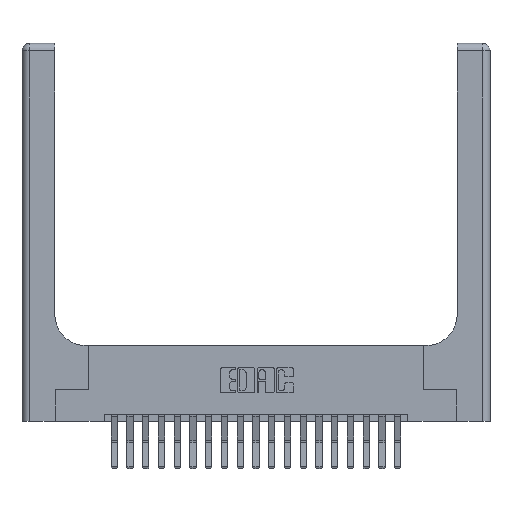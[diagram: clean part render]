
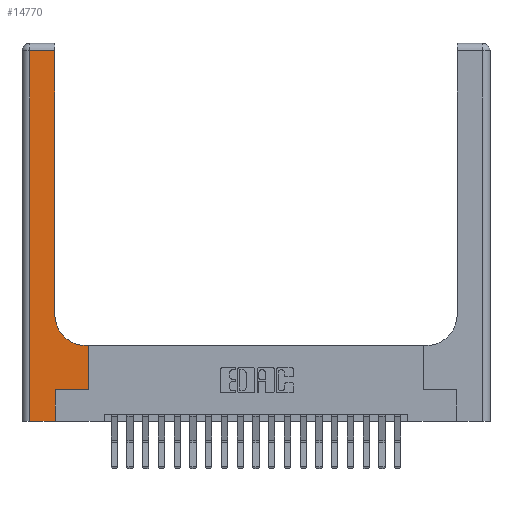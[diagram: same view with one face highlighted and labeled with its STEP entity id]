
A CAD part, top view. The second image highlights one B-rep face of the part: STEP entity #14770.
In plain terms, the highlighted planar face has unit normal (0, 0, 1).
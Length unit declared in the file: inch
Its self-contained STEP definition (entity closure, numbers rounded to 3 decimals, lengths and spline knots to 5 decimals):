
#104 = DIRECTION ( 'NONE',  ( -1., 0., 0. ) ) ;
#171 = AXIS2_PLACEMENT_3D ( 'NONE', #11845, #18023, #13234 ) ;
#428 = AXIS2_PLACEMENT_3D ( 'NONE', #6232, #6744, #3614 ) ;
#624 = PLANE ( 'NONE',  #171 ) ;
#660 = CARTESIAN_POINT ( 'NONE',  ( 0.265, 0., 0.37 ) ) ;
#734 = LINE ( 'NONE', #19692, #10014 ) ;
#1097 = ORIENTED_EDGE ( 'NONE', *, *, #12004, .T. ) ;
#1390 = ORIENTED_EDGE ( 'NONE', *, *, #6338, .T. ) ;
#1741 = CARTESIAN_POINT ( 'NONE',  ( 0.528, 0.6, 0.37 ) ) ;
#2128 = VERTEX_POINT ( 'NONE', #15202 ) ;
#2499 = ORIENTED_EDGE ( 'NONE', *, *, #4910, .T. ) ;
#2816 = ORIENTED_EDGE ( 'NONE', *, *, #12132, .T. ) ;
#3066 = CARTESIAN_POINT ( 'NONE',  ( 0.26, 2.94, 0.37 ) ) ;
#3614 = DIRECTION ( 'NONE',  ( 1., 0., 0. ) ) ;
#3796 = LINE ( 'NONE', #9375, #9843 ) ;
#3816 = ORIENTED_EDGE ( 'NONE', *, *, #19286, .T. ) ;
#4628 = LINE ( 'NONE', #12545, #4862 ) ;
#4636 = LINE ( 'NONE', #17429, #7363 ) ;
#4812 = CARTESIAN_POINT ( 'NONE',  ( 0., 0., 0.37 ) ) ;
#4831 = ORIENTED_EDGE ( 'NONE', *, *, #18948, .T. ) ;
#4835 = DIRECTION ( 'NONE',  ( -1., 0., 0. ) ) ;
#4862 = VECTOR ( 'NONE', #5968, 39.37008 ) ;
#4910 = EDGE_CURVE ( 'NONE', #11582, #2128, #4636, .T. ) ;
#5968 = DIRECTION ( 'NONE',  ( 0., 1., 0. ) ) ;
#6198 = ORIENTED_EDGE ( 'NONE', *, *, #20496, .T. ) ;
#6232 = CARTESIAN_POINT ( 'NONE',  ( 0.51, 0.85, 0.37 ) ) ;
#6338 = EDGE_CURVE ( 'NONE', #17638, #14887, #8106, .T. ) ;
#6652 = VERTEX_POINT ( 'NONE', #9363 ) ;
#6744 = DIRECTION ( 'NONE',  ( 0., 0., -1. ) ) ;
#6790 = LINE ( 'NONE', #19255, #13029 ) ;
#7363 = VECTOR ( 'NONE', #4835, 39.37008 ) ;
#7377 = CARTESIAN_POINT ( 'NONE',  ( 0.265, 0.25, 0.37 ) ) ;
#7416 = EDGE_CURVE ( 'NONE', #7920, #6652, #15059, .T. ) ;
#7920 = VERTEX_POINT ( 'NONE', #18841 ) ;
#8068 = CIRCLE ( 'NONE', #428, 0.25 ) ;
#8106 = LINE ( 'NONE', #11515, #16104 ) ;
#8283 = DIRECTION ( 'NONE',  ( 1., 0., 0. ) ) ;
#9306 = DIRECTION ( 'NONE',  ( 1., 0., 0. ) ) ;
#9363 = CARTESIAN_POINT ( 'NONE',  ( 0.06, 0., 0.37 ) ) ;
#9375 = CARTESIAN_POINT ( 'NONE',  ( 0.265, 0.25, 0.37 ) ) ;
#9843 = VECTOR ( 'NONE', #9306, 39.37008 ) ;
#10014 = VECTOR ( 'NONE', #11834, 39.37008 ) ;
#10081 = VECTOR ( 'NONE', #20060, 39.37008 ) ;
#10682 = CARTESIAN_POINT ( 'NONE',  ( 0.26, 0.85, 0.37 ) ) ;
#10683 = FACE_OUTER_BOUND ( 'NONE', #16678, .T. ) ;
#11515 = CARTESIAN_POINT ( 'NONE',  ( 0.265, 0., 0.37 ) ) ;
#11580 = CARTESIAN_POINT ( 'NONE',  ( 0.06, 3., 0.37 ) ) ;
#11582 = VERTEX_POINT ( 'NONE', #1741 ) ;
#11834 = DIRECTION ( 'NONE',  ( 0., 1., 0. ) ) ;
#11845 = CARTESIAN_POINT ( 'NONE',  ( 0., 3., 0.37 ) ) ;
#12004 = EDGE_CURVE ( 'NONE', #14242, #13864, #4628, .T. ) ;
#12132 = EDGE_CURVE ( 'NONE', #2128, #14242, #8068, .T. ) ;
#12137 = VERTEX_POINT ( 'NONE', #14777 ) ;
#12167 = ORIENTED_EDGE ( 'NONE', *, *, #15923, .T. ) ;
#12545 = CARTESIAN_POINT ( 'NONE',  ( 0.26, 3., 0.37 ) ) ;
#13029 = VECTOR ( 'NONE', #104, 39.37008 ) ;
#13169 = ORIENTED_EDGE ( 'NONE', *, *, #7416, .T. ) ;
#13234 = DIRECTION ( 'NONE',  ( -1., 0., 0. ) ) ;
#13584 = LINE ( 'NONE', #4812, #14093 ) ;
#13864 = VERTEX_POINT ( 'NONE', #3066 ) ;
#14093 = VECTOR ( 'NONE', #8283, 39.37008 ) ;
#14242 = VERTEX_POINT ( 'NONE', #10682 ) ;
#14770 = ADVANCED_FACE ( 'NONE', ( #10683 ), #624, .F. ) ;
#14777 = CARTESIAN_POINT ( 'NONE',  ( 0.528, 0.25, 0.37 ) ) ;
#14887 = VERTEX_POINT ( 'NONE', #7377 ) ;
#15059 = LINE ( 'NONE', #11580, #10081 ) ;
#15202 = CARTESIAN_POINT ( 'NONE',  ( 0.51, 0.6, 0.37 ) ) ;
#15923 = EDGE_CURVE ( 'NONE', #14887, #12137, #3796, .T. ) ;
#16104 = VECTOR ( 'NONE', #16542, 39.37008 ) ;
#16542 = DIRECTION ( 'NONE',  ( 0., 1., 0. ) ) ;
#16678 = EDGE_LOOP ( 'NONE', ( #1097, #6198, #13169, #3816, #1390, #12167, #4831, #2499, #2816 ) ) ;
#17429 = CARTESIAN_POINT ( 'NONE',  ( 0.26, 0.6, 0.37 ) ) ;
#17638 = VERTEX_POINT ( 'NONE', #660 ) ;
#18023 = DIRECTION ( 'NONE',  ( 0., 0., -1. ) ) ;
#18841 = CARTESIAN_POINT ( 'NONE',  ( 0.06, 2.94, 0.37 ) ) ;
#18948 = EDGE_CURVE ( 'NONE', #12137, #11582, #734, .T. ) ;
#19255 = CARTESIAN_POINT ( 'NONE',  ( 0., 2.94, 0.37 ) ) ;
#19286 = EDGE_CURVE ( 'NONE', #6652, #17638, #13584, .T. ) ;
#19692 = CARTESIAN_POINT ( 'NONE',  ( 0.528, 0.25, 0.37 ) ) ;
#20060 = DIRECTION ( 'NONE',  ( 0., -1., 0. ) ) ;
#20496 = EDGE_CURVE ( 'NONE', #13864, #7920, #6790, .T. ) ;
